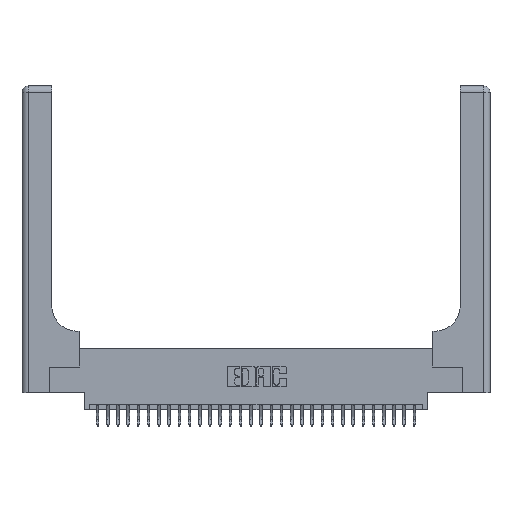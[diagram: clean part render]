
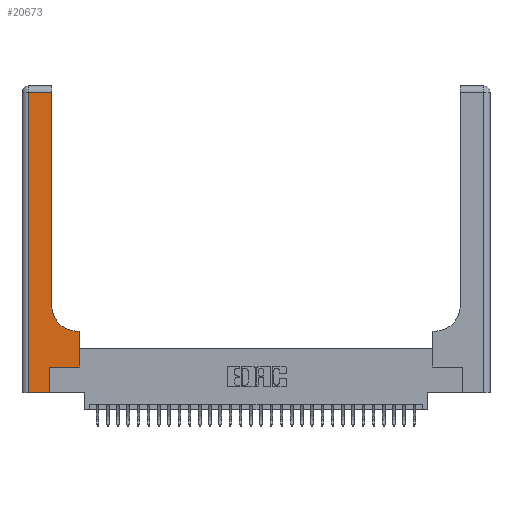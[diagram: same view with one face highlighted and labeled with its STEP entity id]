
A CAD part, top view. The second image highlights one B-rep face of the part: STEP entity #20673.
In plain terms, the highlighted planar face has unit normal (0, 0, 1).
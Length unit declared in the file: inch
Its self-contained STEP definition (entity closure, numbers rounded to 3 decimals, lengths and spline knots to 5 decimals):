
#174 = CARTESIAN_POINT ( 'NONE',  ( 0.06, 2.94, 0.37 ) ) ;
#513 = DIRECTION ( 'NONE',  ( 0., 1., 0. ) ) ;
#683 = DIRECTION ( 'NONE',  ( -1., 0., 0. ) ) ;
#1058 = EDGE_CURVE ( 'NONE', #18786, #13565, #18911, .T. ) ;
#1743 = LINE ( 'NONE', #30279, #26522 ) ;
#2067 = VECTOR ( 'NONE', #21909, 39.37008 ) ;
#2839 = LINE ( 'NONE', #11971, #2067 ) ;
#3462 = CARTESIAN_POINT ( 'NONE',  ( 0.5415, 0.85, 0.37 ) ) ;
#3683 = VERTEX_POINT ( 'NONE', #12152 ) ;
#4376 = CARTESIAN_POINT ( 'NONE',  ( 0.2915, 3., 0.37 ) ) ;
#5005 = FACE_OUTER_BOUND ( 'NONE', #31257, .T. ) ;
#5706 = VECTOR ( 'NONE', #29049, 39.37008 ) ;
#5973 = DIRECTION ( 'NONE',  ( 1., 0., 0. ) ) ;
#8035 = CARTESIAN_POINT ( 'NONE',  ( 0.5585, 0.6, 0.37 ) ) ;
#8853 = ORIENTED_EDGE ( 'NONE', *, *, #11049, .T. ) ;
#8973 = VERTEX_POINT ( 'NONE', #14563 ) ;
#9337 = EDGE_CURVE ( 'NONE', #12426, #8973, #10665, .T. ) ;
#9371 = CARTESIAN_POINT ( 'NONE',  ( 0., 0., 0.37 ) ) ;
#9604 = DIRECTION ( 'NONE',  ( -1., 0., 0. ) ) ;
#9719 = VECTOR ( 'NONE', #24279, 39.37008 ) ;
#10361 = VECTOR ( 'NONE', #31618, 39.37008 ) ;
#10665 = CIRCLE ( 'NONE', #24282, 0.25 ) ;
#10686 = VERTEX_POINT ( 'NONE', #21720 ) ;
#11049 = EDGE_CURVE ( 'NONE', #13565, #11566, #20558, .T. ) ;
#11153 = ORIENTED_EDGE ( 'NONE', *, *, #23176, .T. ) ;
#11566 = VERTEX_POINT ( 'NONE', #20350 ) ;
#11588 = ORIENTED_EDGE ( 'NONE', *, *, #12765, .T. ) ;
#11948 = CARTESIAN_POINT ( 'NONE',  ( 0.2915, 0.6, 0.37 ) ) ;
#11971 = CARTESIAN_POINT ( 'NONE',  ( 0.5585, 0.25, 0.37 ) ) ;
#12152 = CARTESIAN_POINT ( 'NONE',  ( 0.2915, 2.94, 0.37 ) ) ;
#12426 = VERTEX_POINT ( 'NONE', #14025 ) ;
#12723 = CARTESIAN_POINT ( 'NONE',  ( 0.06, 0., 0.37 ) ) ;
#12765 = EDGE_CURVE ( 'NONE', #11566, #10686, #19311, .T. ) ;
#12923 = DIRECTION ( 'NONE',  ( 1., 0., 0. ) ) ;
#13565 = VERTEX_POINT ( 'NONE', #15795 ) ;
#14025 = CARTESIAN_POINT ( 'NONE',  ( 0.5415, 0.6, 0.37 ) ) ;
#14266 = PLANE ( 'NONE',  #29808 ) ;
#14563 = CARTESIAN_POINT ( 'NONE',  ( 0.2915, 0.85, 0.37 ) ) ;
#14687 = EDGE_CURVE ( 'NONE', #10686, #16787, #2839, .T. ) ;
#15795 = CARTESIAN_POINT ( 'NONE',  ( 0.269, 0., 0.37 ) ) ;
#16580 = ORIENTED_EDGE ( 'NONE', *, *, #1058, .T. ) ;
#16787 = VERTEX_POINT ( 'NONE', #8035 ) ;
#16848 = DIRECTION ( 'NONE',  ( 0., 1., 0. ) ) ;
#16962 = CARTESIAN_POINT ( 'NONE',  ( 0., 3., 0.37 ) ) ;
#18786 = VERTEX_POINT ( 'NONE', #12723 ) ;
#18911 = LINE ( 'NONE', #9371, #5706 ) ;
#19311 = LINE ( 'NONE', #25207, #30775 ) ;
#19386 = ORIENTED_EDGE ( 'NONE', *, *, #14687, .T. ) ;
#20350 = CARTESIAN_POINT ( 'NONE',  ( 0.269, 0.25, 0.37 ) ) ;
#20558 = LINE ( 'NONE', #22864, #26305 ) ;
#20673 = ADVANCED_FACE ( 'NONE', ( #5005 ), #14266, .F. ) ;
#20812 = DIRECTION ( 'NONE',  ( 0., 0., -1. ) ) ;
#21621 = ORIENTED_EDGE ( 'NONE', *, *, #31389, .T. ) ;
#21720 = CARTESIAN_POINT ( 'NONE',  ( 0.5585, 0.25, 0.37 ) ) ;
#21909 = DIRECTION ( 'NONE',  ( 0., 1., 0. ) ) ;
#22864 = CARTESIAN_POINT ( 'NONE',  ( 0.269, 0., 0.37 ) ) ;
#23176 = EDGE_CURVE ( 'NONE', #3683, #27219, #1743, .T. ) ;
#23988 = EDGE_CURVE ( 'NONE', #8973, #3683, #30188, .T. ) ;
#24211 = ORIENTED_EDGE ( 'NONE', *, *, #23988, .T. ) ;
#24279 = DIRECTION ( 'NONE',  ( 0., -1., 0. ) ) ;
#24282 = AXIS2_PLACEMENT_3D ( 'NONE', #3462, #20812, #5973 ) ;
#24403 = DIRECTION ( 'NONE',  ( 0., 0., -1. ) ) ;
#25207 = CARTESIAN_POINT ( 'NONE',  ( 0.269, 0.25, 0.37 ) ) ;
#26305 = VECTOR ( 'NONE', #513, 39.37008 ) ;
#26522 = VECTOR ( 'NONE', #683, 39.37008 ) ;
#27219 = VERTEX_POINT ( 'NONE', #174 ) ;
#27689 = EDGE_CURVE ( 'NONE', #16787, #12426, #29978, .T. ) ;
#29049 = DIRECTION ( 'NONE',  ( 1., 0., 0. ) ) ;
#29420 = VECTOR ( 'NONE', #16848, 39.37008 ) ;
#29808 = AXIS2_PLACEMENT_3D ( 'NONE', #16962, #24403, #9604 ) ;
#29978 = LINE ( 'NONE', #11948, #10361 ) ;
#30104 = LINE ( 'NONE', #31637, #9719 ) ;
#30106 = ORIENTED_EDGE ( 'NONE', *, *, #27689, .T. ) ;
#30188 = LINE ( 'NONE', #4376, #29420 ) ;
#30279 = CARTESIAN_POINT ( 'NONE',  ( 0., 2.94, 0.37 ) ) ;
#30775 = VECTOR ( 'NONE', #12923, 39.37008 ) ;
#31257 = EDGE_LOOP ( 'NONE', ( #24211, #11153, #21621, #16580, #8853, #11588, #19386, #30106, #31675 ) ) ;
#31389 = EDGE_CURVE ( 'NONE', #27219, #18786, #30104, .T. ) ;
#31618 = DIRECTION ( 'NONE',  ( -1., 0., 0. ) ) ;
#31637 = CARTESIAN_POINT ( 'NONE',  ( 0.06, 3., 0.37 ) ) ;
#31675 = ORIENTED_EDGE ( 'NONE', *, *, #9337, .T. ) ;
